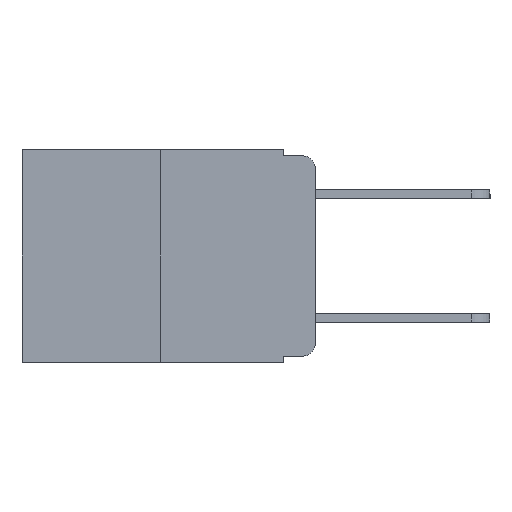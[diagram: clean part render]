
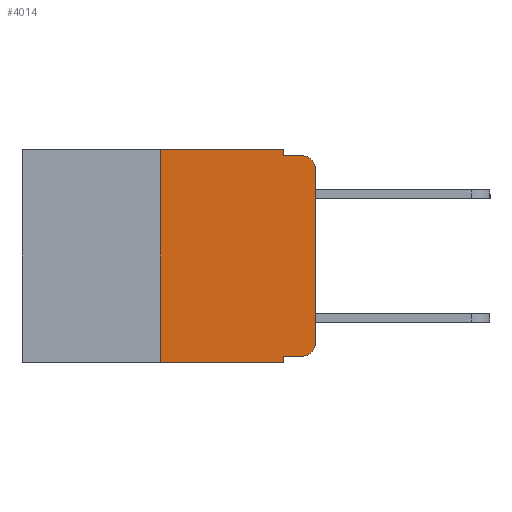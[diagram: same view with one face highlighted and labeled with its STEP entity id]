
A CAD part, left-side view. The second image highlights one B-rep face of the part: STEP entity #4014.
In plain terms, the highlighted planar face has unit normal (-1, 0, 0).
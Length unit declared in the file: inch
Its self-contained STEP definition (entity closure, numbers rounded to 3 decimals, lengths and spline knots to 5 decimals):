
#292 = VECTOR ( 'NONE', #8722, 39.37008 ) ;
#416 = AXIS2_PLACEMENT_3D ( 'NONE', #7335, #2500, #8030 ) ;
#676 = ORIENTED_EDGE ( 'NONE', *, *, #8110, .T. ) ;
#733 = PLANE ( 'NONE',  #4022 ) ;
#900 = CIRCLE ( 'NONE', #416, 0.02 ) ;
#1099 = LINE ( 'NONE', #2386, #5104 ) ;
#1117 = EDGE_CURVE ( 'NONE', #6850, #2836, #8784, .T. ) ;
#1376 = EDGE_LOOP ( 'NONE', ( #4120, #1957, #9720, #8211, #4386, #2963, #676, #6588, #8561, #6791 ) ) ;
#1757 = AXIS2_PLACEMENT_3D ( 'NONE', #8884, #8864, #8853 ) ;
#1922 = CARTESIAN_POINT ( 'NONE',  ( 0., 0.25, 0. ) ) ;
#1957 = ORIENTED_EDGE ( 'NONE', *, *, #8828, .T. ) ;
#2386 = CARTESIAN_POINT ( 'NONE',  ( 0., 0.051, 0. ) ) ;
#2400 = DIRECTION ( 'NONE',  ( 0., 0., -1. ) ) ;
#2500 = DIRECTION ( 'NONE',  ( -1., 0., 0. ) ) ;
#2504 = VERTEX_POINT ( 'NONE', #9086 ) ;
#2658 = LINE ( 'NONE', #6016, #292 ) ;
#2836 = VERTEX_POINT ( 'NONE', #8468 ) ;
#2963 = ORIENTED_EDGE ( 'NONE', *, *, #6123, .F. ) ;
#3136 = CARTESIAN_POINT ( 'NONE',  ( 0., 0.051, -0.01 ) ) ;
#3171 = VECTOR ( 'NONE', #8772, 39.37008 ) ;
#3287 = VERTEX_POINT ( 'NONE', #3601 ) ;
#3462 = DIRECTION ( 'NONE',  ( 0., -1., 0. ) ) ;
#3601 = CARTESIAN_POINT ( 'NONE',  ( 0., 0.051, -0.343 ) ) ;
#3807 = VECTOR ( 'NONE', #9338, 39.37008 ) ;
#3871 = CARTESIAN_POINT ( 'NONE',  ( 0., 0.051, -0.333 ) ) ;
#4014 = ADVANCED_FACE ( 'NONE', ( #8599 ), #733, .F. ) ;
#4022 = AXIS2_PLACEMENT_3D ( 'NONE', #7091, #8002, #9041 ) ;
#4120 = ORIENTED_EDGE ( 'NONE', *, *, #8904, .T. ) ;
#4386 = ORIENTED_EDGE ( 'NONE', *, *, #7521, .F. ) ;
#4530 = VERTEX_POINT ( 'NONE', #5735 ) ;
#4646 = CARTESIAN_POINT ( 'NONE',  ( 0., 0., -0.313 ) ) ;
#4678 = VERTEX_POINT ( 'NONE', #8307 ) ;
#4954 = LINE ( 'NONE', #8088, #8370 ) ;
#5056 = VECTOR ( 'NONE', #3462, 39.37008 ) ;
#5104 = VECTOR ( 'NONE', #2400, 39.37008 ) ;
#5137 = CARTESIAN_POINT ( 'NONE',  ( 0., 0.25, -0.343 ) ) ;
#5271 = DIRECTION ( 'NONE',  ( 0., -1., 0. ) ) ;
#5382 = CIRCLE ( 'NONE', #1757, 0.02 ) ;
#5514 = VERTEX_POINT ( 'NONE', #5137 ) ;
#5735 = CARTESIAN_POINT ( 'NONE',  ( 0., 0.02, -0.333 ) ) ;
#5980 = EDGE_CURVE ( 'NONE', #4530, #6973, #5382, .T. ) ;
#5982 = DIRECTION ( 'NONE',  ( 0., 0., 1. ) ) ;
#6016 = CARTESIAN_POINT ( 'NONE',  ( 0., 0.051, 0. ) ) ;
#6123 = EDGE_CURVE ( 'NONE', #5514, #6517, #4954, .T. ) ;
#6324 = LINE ( 'NONE', #7547, #9337 ) ;
#6517 = VERTEX_POINT ( 'NONE', #1922 ) ;
#6584 = EDGE_CURVE ( 'NONE', #8507, #3287, #1099, .T. ) ;
#6588 = ORIENTED_EDGE ( 'NONE', *, *, #6584, .F. ) ;
#6791 = ORIENTED_EDGE ( 'NONE', *, *, #5980, .T. ) ;
#6850 = VERTEX_POINT ( 'NONE', #3136 ) ;
#6973 = VERTEX_POINT ( 'NONE', #4646 ) ;
#7091 = CARTESIAN_POINT ( 'NONE',  ( 0., 0.473, 0. ) ) ;
#7335 = CARTESIAN_POINT ( 'NONE',  ( 0., 0.02, -0.03 ) ) ;
#7434 = CARTESIAN_POINT ( 'NONE',  ( 0., 0.051, -0.01 ) ) ;
#7514 = EDGE_CURVE ( 'NONE', #8507, #4530, #9508, .T. ) ;
#7521 = EDGE_CURVE ( 'NONE', #6517, #2504, #6324, .T. ) ;
#7547 = CARTESIAN_POINT ( 'NONE',  ( 0., 0.473, 0. ) ) ;
#7681 = LINE ( 'NONE', #9357, #3171 ) ;
#7972 = LINE ( 'NONE', #9821, #9312 ) ;
#8002 = DIRECTION ( 'NONE',  ( 1., 0., 0. ) ) ;
#8030 = DIRECTION ( 'NONE',  ( 0., 0., -1. ) ) ;
#8088 = CARTESIAN_POINT ( 'NONE',  ( 0., 0.25, 0. ) ) ;
#8103 = DIRECTION ( 'NONE',  ( 0., 0., 1. ) ) ;
#8110 = EDGE_CURVE ( 'NONE', #5514, #3287, #7681, .T. ) ;
#8211 = ORIENTED_EDGE ( 'NONE', *, *, #8933, .F. ) ;
#8307 = CARTESIAN_POINT ( 'NONE',  ( 0., 0., -0.03 ) ) ;
#8370 = VECTOR ( 'NONE', #8103, 39.37008 ) ;
#8468 = CARTESIAN_POINT ( 'NONE',  ( 0., 0.02, -0.01 ) ) ;
#8507 = VERTEX_POINT ( 'NONE', #3871 ) ;
#8561 = ORIENTED_EDGE ( 'NONE', *, *, #7514, .T. ) ;
#8599 = FACE_OUTER_BOUND ( 'NONE', #1376, .T. ) ;
#8722 = DIRECTION ( 'NONE',  ( 0., 0., -1. ) ) ;
#8756 = CARTESIAN_POINT ( 'NONE',  ( 0., 0.051, -0.333 ) ) ;
#8772 = DIRECTION ( 'NONE',  ( 0., -1., 0. ) ) ;
#8784 = LINE ( 'NONE', #7434, #5056 ) ;
#8828 = EDGE_CURVE ( 'NONE', #4678, #2836, #900, .T. ) ;
#8853 = DIRECTION ( 'NONE',  ( 0., 0., -1. ) ) ;
#8864 = DIRECTION ( 'NONE',  ( -1., 0., 0. ) ) ;
#8884 = CARTESIAN_POINT ( 'NONE',  ( 0., 0.02, -0.313 ) ) ;
#8904 = EDGE_CURVE ( 'NONE', #6973, #4678, #7972, .T. ) ;
#8933 = EDGE_CURVE ( 'NONE', #2504, #6850, #2658, .T. ) ;
#9041 = DIRECTION ( 'NONE',  ( 0., 0., -1. ) ) ;
#9086 = CARTESIAN_POINT ( 'NONE',  ( 0., 0.051, 0. ) ) ;
#9312 = VECTOR ( 'NONE', #5982, 39.37008 ) ;
#9337 = VECTOR ( 'NONE', #5271, 39.37008 ) ;
#9338 = DIRECTION ( 'NONE',  ( 0., -1., 0. ) ) ;
#9357 = CARTESIAN_POINT ( 'NONE',  ( 0., 0.473, -0.343 ) ) ;
#9508 = LINE ( 'NONE', #8756, #3807 ) ;
#9720 = ORIENTED_EDGE ( 'NONE', *, *, #1117, .F. ) ;
#9821 = CARTESIAN_POINT ( 'NONE',  ( 0., 0., 0. ) ) ;
